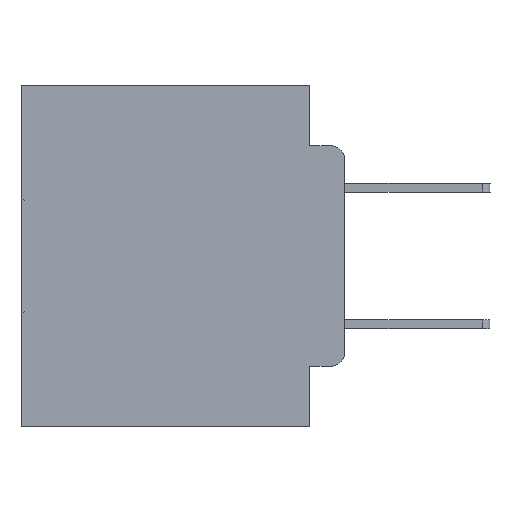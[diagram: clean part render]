
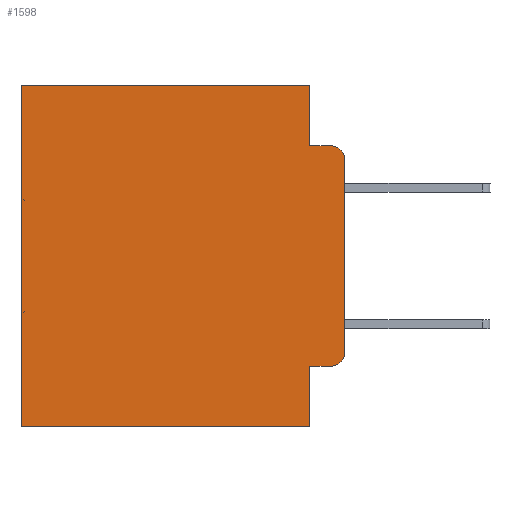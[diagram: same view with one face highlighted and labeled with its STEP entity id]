
A CAD part, left-side view. The second image highlights one B-rep face of the part: STEP entity #1598.
In plain terms, the highlighted planar face has unit normal (-1, 0, 0).
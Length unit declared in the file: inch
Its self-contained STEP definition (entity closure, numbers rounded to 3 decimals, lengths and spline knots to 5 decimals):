
#569 = ORIENTED_EDGE ( 'NONE', *, *, #30513, .T. ) ;
#840 = CARTESIAN_POINT ( 'NONE',  ( 0.298, 0., 0. ) ) ;
#1137 = CARTESIAN_POINT ( 'NONE',  ( 0.298, 0.051, -0.5 ) ) ;
#1140 = EDGE_CURVE ( 'NONE', #24782, #6577, #11508, .T. ) ;
#1598 = ADVANCED_FACE ( 'NONE', ( #5490 ), #24417, .F. ) ;
#1678 = CARTESIAN_POINT ( 'NONE',  ( 0.298, 0.02, -0.4115 ) ) ;
#1684 = CIRCLE ( 'NONE', #3280, 0.02 ) ;
#1909 = CARTESIAN_POINT ( 'NONE',  ( 0.298, 0.473, 0. ) ) ;
#2244 = VECTOR ( 'NONE', #32505, 39.37008 ) ;
#2263 = EDGE_CURVE ( 'NONE', #24844, #6388, #5839, .T. ) ;
#2857 = VERTEX_POINT ( 'NONE', #11282 ) ;
#3280 = AXIS2_PLACEMENT_3D ( 'NONE', #28044, #12933, #30587 ) ;
#3613 = CARTESIAN_POINT ( 'NONE',  ( 0.298, 0.02, -0.3915 ) ) ;
#3774 = ORIENTED_EDGE ( 'NONE', *, *, #28074, .T. ) ;
#4105 = CARTESIAN_POINT ( 'NONE',  ( 0.298, 0.02, -0.0885 ) ) ;
#4403 = DIRECTION ( 'NONE',  ( 0., -1., 0. ) ) ;
#4684 = CARTESIAN_POINT ( 'NONE',  ( 0.298, 0.051, -0.0885 ) ) ;
#5203 = VERTEX_POINT ( 'NONE', #8357 ) ;
#5422 = ORIENTED_EDGE ( 'NONE', *, *, #6998, .F. ) ;
#5490 = FACE_OUTER_BOUND ( 'NONE', #8074, .T. ) ;
#5839 = LINE ( 'NONE', #9429, #31942 ) ;
#6222 = DIRECTION ( 'NONE',  ( 0., 0., -1. ) ) ;
#6388 = VERTEX_POINT ( 'NONE', #28459 ) ;
#6444 = CARTESIAN_POINT ( 'NONE',  ( 0.298, 0.051, -0.4115 ) ) ;
#6484 = CARTESIAN_POINT ( 'NONE',  ( 0.298, 0.051, -0.0885 ) ) ;
#6577 = VERTEX_POINT ( 'NONE', #1678 ) ;
#6998 = EDGE_CURVE ( 'NONE', #24782, #17015, #18277, .T. ) ;
#7007 = ORIENTED_EDGE ( 'NONE', *, *, #1140, .T. ) ;
#7044 = ORIENTED_EDGE ( 'NONE', *, *, #23577, .F. ) ;
#7897 = VERTEX_POINT ( 'NONE', #1909 ) ;
#8009 = DIRECTION ( 'NONE',  ( 1., 0., 0. ) ) ;
#8074 = EDGE_LOOP ( 'NONE', ( #12965, #29551, #17755, #11791, #3774, #569, #7044, #5422, #7007, #24778 ) ) ;
#8357 = CARTESIAN_POINT ( 'NONE',  ( 0.298, 0.051, 0. ) ) ;
#9429 = CARTESIAN_POINT ( 'NONE',  ( 0.298, 0., 0. ) ) ;
#10428 = CARTESIAN_POINT ( 'NONE',  ( 0.298, 0., -0.1085 ) ) ;
#11032 = DIRECTION ( 'NONE',  ( 0., 1., 0. ) ) ;
#11095 = DIRECTION ( 'NONE',  ( 0., 0., -1. ) ) ;
#11282 = CARTESIAN_POINT ( 'NONE',  ( 0.298, 0.473, -0.5 ) ) ;
#11456 = VECTOR ( 'NONE', #28670, 39.37008 ) ;
#11508 = LINE ( 'NONE', #6444, #12314 ) ;
#11791 = ORIENTED_EDGE ( 'NONE', *, *, #21430, .F. ) ;
#12314 = VECTOR ( 'NONE', #4403, 39.37008 ) ;
#12870 = CARTESIAN_POINT ( 'NONE',  ( 0.298, 0.051, 0. ) ) ;
#12933 = DIRECTION ( 'NONE',  ( -1., 0., 0. ) ) ;
#12965 = ORIENTED_EDGE ( 'NONE', *, *, #2263, .F. ) ;
#14856 = AXIS2_PLACEMENT_3D ( 'NONE', #18152, #8009, #24531 ) ;
#14977 = LINE ( 'NONE', #31167, #20900 ) ;
#15555 = VECTOR ( 'NONE', #11032, 39.37008 ) ;
#15739 = CIRCLE ( 'NONE', #27179, 0.02 ) ;
#15962 = VERTEX_POINT ( 'NONE', #6484 ) ;
#16041 = VERTEX_POINT ( 'NONE', #4105 ) ;
#16125 = CARTESIAN_POINT ( 'NONE',  ( 0.298, 0.051, 0. ) ) ;
#16964 = EDGE_CURVE ( 'NONE', #6577, #6388, #15739, .T. ) ;
#17015 = VERTEX_POINT ( 'NONE', #1137 ) ;
#17490 = VECTOR ( 'NONE', #19182, 39.37008 ) ;
#17740 = CARTESIAN_POINT ( 'NONE',  ( 0.298, 0.051, -0.4115 ) ) ;
#17755 = ORIENTED_EDGE ( 'NONE', *, *, #27760, .F. ) ;
#18152 = CARTESIAN_POINT ( 'NONE',  ( 0.298, 0., 0. ) ) ;
#18277 = LINE ( 'NONE', #12870, #17490 ) ;
#19182 = DIRECTION ( 'NONE',  ( 0., 0., -1. ) ) ;
#19893 = CARTESIAN_POINT ( 'NONE',  ( 0.298, 0., -0.5 ) ) ;
#20900 = VECTOR ( 'NONE', #11095, 39.37008 ) ;
#21402 = DIRECTION ( 'NONE',  ( -1., 0., 0. ) ) ;
#21430 = EDGE_CURVE ( 'NONE', #5203, #15962, #31578, .T. ) ;
#22556 = LINE ( 'NONE', #19893, #2244 ) ;
#23430 = VECTOR ( 'NONE', #30056, 39.37008 ) ;
#23577 = EDGE_CURVE ( 'NONE', #17015, #2857, #22556, .T. ) ;
#24417 = PLANE ( 'NONE',  #14856 ) ;
#24531 = DIRECTION ( 'NONE',  ( 0., 0., -1. ) ) ;
#24778 = ORIENTED_EDGE ( 'NONE', *, *, #16964, .T. ) ;
#24782 = VERTEX_POINT ( 'NONE', #17740 ) ;
#24844 = VERTEX_POINT ( 'NONE', #10428 ) ;
#26072 = EDGE_CURVE ( 'NONE', #24844, #16041, #1684, .T. ) ;
#26272 = DIRECTION ( 'NONE',  ( 0., 0., -1. ) ) ;
#27179 = AXIS2_PLACEMENT_3D ( 'NONE', #3613, #21402, #6222 ) ;
#27760 = EDGE_CURVE ( 'NONE', #15962, #16041, #30161, .T. ) ;
#28044 = CARTESIAN_POINT ( 'NONE',  ( 0.298, 0.02, -0.1085 ) ) ;
#28074 = EDGE_CURVE ( 'NONE', #5203, #7897, #28167, .T. ) ;
#28167 = LINE ( 'NONE', #840, #15555 ) ;
#28459 = CARTESIAN_POINT ( 'NONE',  ( 0.298, 0., -0.3915 ) ) ;
#28670 = DIRECTION ( 'NONE',  ( 0., 0., -1. ) ) ;
#29551 = ORIENTED_EDGE ( 'NONE', *, *, #26072, .T. ) ;
#30056 = DIRECTION ( 'NONE',  ( 0., -1., 0. ) ) ;
#30161 = LINE ( 'NONE', #4684, #23430 ) ;
#30513 = EDGE_CURVE ( 'NONE', #7897, #2857, #14977, .T. ) ;
#30587 = DIRECTION ( 'NONE',  ( 0., 0., -1. ) ) ;
#31167 = CARTESIAN_POINT ( 'NONE',  ( 0.298, 0.473, 0. ) ) ;
#31578 = LINE ( 'NONE', #16125, #11456 ) ;
#31942 = VECTOR ( 'NONE', #26272, 39.37008 ) ;
#32505 = DIRECTION ( 'NONE',  ( 0., 1., 0. ) ) ;
